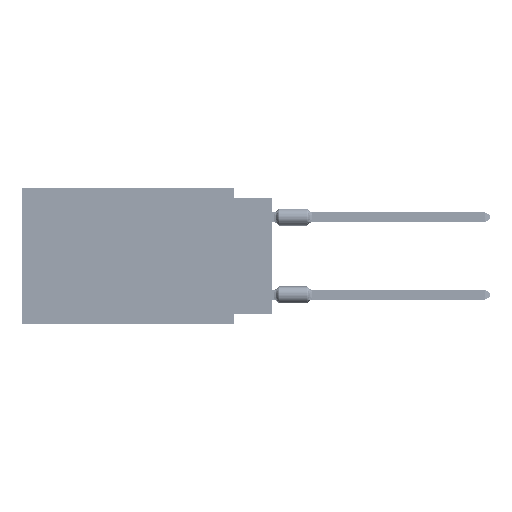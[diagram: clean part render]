
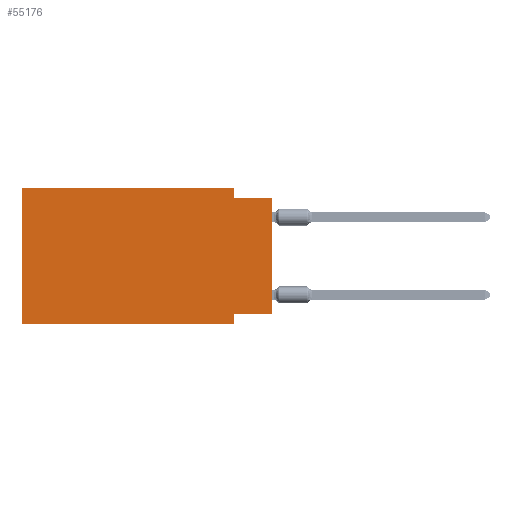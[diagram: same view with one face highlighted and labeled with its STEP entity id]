
A CAD part, left-side view. The second image highlights one B-rep face of the part: STEP entity #55176.
In plain terms, the highlighted planar face has unit normal (-1, 0, 0).
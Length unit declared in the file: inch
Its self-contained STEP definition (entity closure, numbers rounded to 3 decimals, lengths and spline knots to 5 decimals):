
#142 = VERTEX_POINT ( 'NONE', #25851 ) ;
#2327 = EDGE_CURVE ( 'NONE', #56208, #27061, #70556, .T. ) ;
#2555 = CARTESIAN_POINT ( 'NONE',  ( 0., 0., -0.025 ) ) ;
#8261 = AXIS2_PLACEMENT_3D ( 'NONE', #49374, #69696, #76044 ) ;
#8629 = EDGE_CURVE ( 'NONE', #13653, #27061, #61704, .T. ) ;
#12011 = VERTEX_POINT ( 'NONE', #32356 ) ;
#13188 = VECTOR ( 'NONE', #24107, 39.37008 ) ;
#13653 = VERTEX_POINT ( 'NONE', #55072 ) ;
#16610 = VECTOR ( 'NONE', #67128, 39.37008 ) ;
#17193 = CARTESIAN_POINT ( 'NONE',  ( 0., 0.1, -0.325 ) ) ;
#19006 = DIRECTION ( 'NONE',  ( 0., 0., -1. ) ) ;
#19420 = DIRECTION ( 'NONE',  ( 0., -1., 0. ) ) ;
#20559 = CARTESIAN_POINT ( 'NONE',  ( 0., 0., -0.325 ) ) ;
#20762 = CARTESIAN_POINT ( 'NONE',  ( 0., 0., -0.325 ) ) ;
#21866 = FACE_OUTER_BOUND ( 'NONE', #81010, .T. ) ;
#21918 = VERTEX_POINT ( 'NONE', #17193 ) ;
#24107 = DIRECTION ( 'NONE',  ( 0., 0., 1. ) ) ;
#24790 = ORIENTED_EDGE ( 'NONE', *, *, #32587, .F. ) ;
#25689 = VECTOR ( 'NONE', #75237, 39.37008 ) ;
#25851 = CARTESIAN_POINT ( 'NONE',  ( 0., 0.1, 0. ) ) ;
#26232 = LINE ( 'NONE', #88514, #70535 ) ;
#27061 = VERTEX_POINT ( 'NONE', #2555 ) ;
#27721 = CARTESIAN_POINT ( 'NONE',  ( 0., 0.645, 0. ) ) ;
#27983 = DIRECTION ( 'NONE',  ( 0., 1., 0. ) ) ;
#30439 = VECTOR ( 'NONE', #86810, 39.37008 ) ;
#32356 = CARTESIAN_POINT ( 'NONE',  ( 0., 0.645, -0.35 ) ) ;
#32587 = EDGE_CURVE ( 'NONE', #56208, #21918, #47827, .T. ) ;
#32974 = LINE ( 'NONE', #81264, #70288 ) ;
#40496 = CARTESIAN_POINT ( 'NONE',  ( 0., 0.1, 0. ) ) ;
#41091 = EDGE_CURVE ( 'NONE', #12011, #72545, #32974, .T. ) ;
#43601 = DIRECTION ( 'NONE',  ( 0., -1., 0. ) ) ;
#45233 = EDGE_CURVE ( 'NONE', #21918, #72545, #26232, .T. ) ;
#46013 = CARTESIAN_POINT ( 'NONE',  ( 0., 0.1, -0.35 ) ) ;
#47765 = ORIENTED_EDGE ( 'NONE', *, *, #45233, .F. ) ;
#47827 = LINE ( 'NONE', #20762, #49609 ) ;
#48908 = CARTESIAN_POINT ( 'NONE',  ( 0., 0.645, 0. ) ) ;
#49374 = CARTESIAN_POINT ( 'NONE',  ( 0., 0.645, 0. ) ) ;
#49609 = VECTOR ( 'NONE', #27983, 39.37008 ) ;
#55072 = CARTESIAN_POINT ( 'NONE',  ( 0., 0.1, -0.025 ) ) ;
#55176 = ADVANCED_FACE ( 'NONE', ( #21866 ), #62041, .F. ) ;
#56208 = VERTEX_POINT ( 'NONE', #20559 ) ;
#58520 = EDGE_CURVE ( 'NONE', #82754, #142, #70669, .T. ) ;
#61704 = LINE ( 'NONE', #89266, #16610 ) ;
#62041 = PLANE ( 'NONE',  #8261 ) ;
#63775 = CARTESIAN_POINT ( 'NONE',  ( 0., 0., 0. ) ) ;
#65061 = ORIENTED_EDGE ( 'NONE', *, *, #2327, .T. ) ;
#66971 = ORIENTED_EDGE ( 'NONE', *, *, #58520, .F. ) ;
#67128 = DIRECTION ( 'NONE',  ( 0., -1., 0. ) ) ;
#69268 = VECTOR ( 'NONE', #43601, 39.37008 ) ;
#69696 = DIRECTION ( 'NONE',  ( 1., 0., 0. ) ) ;
#70288 = VECTOR ( 'NONE', #19420, 39.37008 ) ;
#70535 = VECTOR ( 'NONE', #19006, 39.37008 ) ;
#70556 = LINE ( 'NONE', #63775, #30439 ) ;
#70669 = LINE ( 'NONE', #77005, #69268 ) ;
#72545 = VERTEX_POINT ( 'NONE', #46013 ) ;
#73714 = ORIENTED_EDGE ( 'NONE', *, *, #8629, .F. ) ;
#74792 = LINE ( 'NONE', #40496, #25689 ) ;
#75111 = ORIENTED_EDGE ( 'NONE', *, *, #41091, .T. ) ;
#75237 = DIRECTION ( 'NONE',  ( 0., 0., -1. ) ) ;
#76044 = DIRECTION ( 'NONE',  ( 0., 0., -1. ) ) ;
#77005 = CARTESIAN_POINT ( 'NONE',  ( 0., 0.645, 0. ) ) ;
#77790 = LINE ( 'NONE', #48908, #13188 ) ;
#79944 = EDGE_CURVE ( 'NONE', #142, #13653, #74792, .T. ) ;
#80870 = ORIENTED_EDGE ( 'NONE', *, *, #83999, .F. ) ;
#81010 = EDGE_LOOP ( 'NONE', ( #65061, #73714, #88274, #66971, #80870, #75111, #47765, #24790 ) ) ;
#81264 = CARTESIAN_POINT ( 'NONE',  ( 0., 0.645, -0.35 ) ) ;
#82754 = VERTEX_POINT ( 'NONE', #27721 ) ;
#83999 = EDGE_CURVE ( 'NONE', #12011, #82754, #77790, .T. ) ;
#86810 = DIRECTION ( 'NONE',  ( 0., 0., 1. ) ) ;
#88274 = ORIENTED_EDGE ( 'NONE', *, *, #79944, .F. ) ;
#88514 = CARTESIAN_POINT ( 'NONE',  ( 0., 0.1, -0.35 ) ) ;
#89266 = CARTESIAN_POINT ( 'NONE',  ( 0., 0., -0.025 ) ) ;
